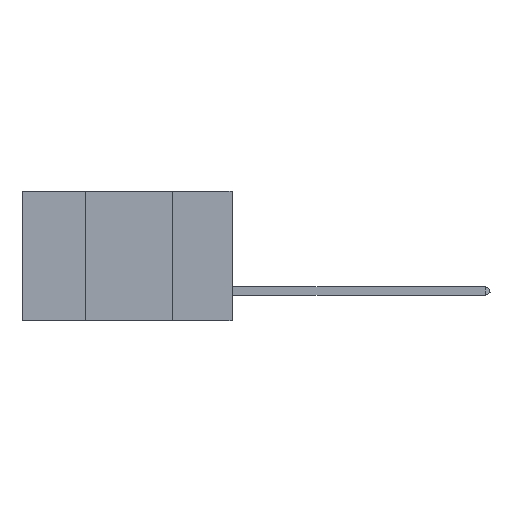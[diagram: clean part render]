
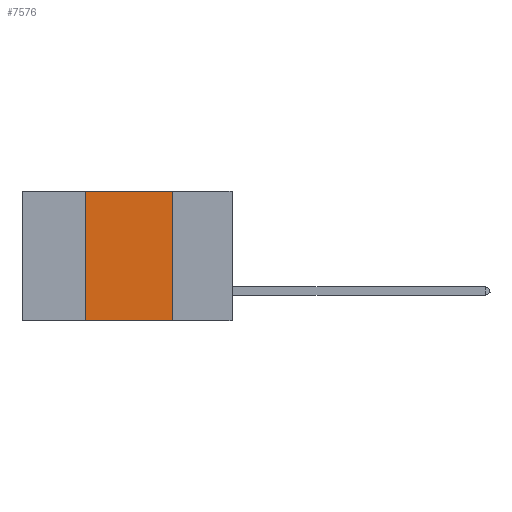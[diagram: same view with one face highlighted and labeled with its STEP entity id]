
A CAD part, left-side view. The second image highlights one B-rep face of the part: STEP entity #7576.
In plain terms, the highlighted planar face has unit normal (-1, 0, 0).
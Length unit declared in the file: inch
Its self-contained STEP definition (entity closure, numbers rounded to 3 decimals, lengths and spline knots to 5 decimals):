
#1481 = DIRECTION ( 'NONE',  ( 0., -1., 0. ) ) ;
#2502 = VECTOR ( 'NONE', #1481, 39.37008 ) ;
#2817 = AXIS2_PLACEMENT_3D ( 'NONE', #18901, #9500, #28714 ) ;
#4020 = LINE ( 'NONE', #27157, #8464 ) ;
#4046 = CARTESIAN_POINT ( 'NONE',  ( 0., 0.17, 0. ) ) ;
#4150 = EDGE_CURVE ( 'NONE', #23712, #28353, #4020, .T. ) ;
#4192 = EDGE_CURVE ( 'NONE', #16608, #23712, #28757, .T. ) ;
#5311 = CARTESIAN_POINT ( 'NONE',  ( 0., 0.6, 0. ) ) ;
#7089 = ORIENTED_EDGE ( 'NONE', *, *, #12730, .F. ) ;
#7200 = PLANE ( 'NONE',  #2817 ) ;
#7576 = ADVANCED_FACE ( 'NONE', ( #10854 ), #7200, .F. ) ;
#7782 = LINE ( 'NONE', #14104, #9268 ) ;
#8464 = VECTOR ( 'NONE', #20046, 39.37008 ) ;
#8812 = CARTESIAN_POINT ( 'NONE',  ( 0., 0.42, -0.37 ) ) ;
#9268 = VECTOR ( 'NONE', #13898, 39.37008 ) ;
#9500 = DIRECTION ( 'NONE',  ( 1., 0., 0. ) ) ;
#9719 = CARTESIAN_POINT ( 'NONE',  ( 0., 0.17, -0.37 ) ) ;
#10376 = ORIENTED_EDGE ( 'NONE', *, *, #4150, .F. ) ;
#10854 = FACE_OUTER_BOUND ( 'NONE', #30782, .T. ) ;
#12133 = DIRECTION ( 'NONE',  ( 0., -1., 0. ) ) ;
#12730 = EDGE_CURVE ( 'NONE', #28231, #16608, #7782, .T. ) ;
#13898 = DIRECTION ( 'NONE',  ( 0., 0., 1. ) ) ;
#14104 = CARTESIAN_POINT ( 'NONE',  ( 0., 0.42, 0. ) ) ;
#14160 = EDGE_CURVE ( 'NONE', #28231, #28353, #26838, .T. ) ;
#16608 = VERTEX_POINT ( 'NONE', #20420 ) ;
#18511 = CARTESIAN_POINT ( 'NONE',  ( 0., 0.6, -0.37 ) ) ;
#18901 = CARTESIAN_POINT ( 'NONE',  ( 0., 0.6, 0. ) ) ;
#20046 = DIRECTION ( 'NONE',  ( 0., 0., -1. ) ) ;
#20420 = CARTESIAN_POINT ( 'NONE',  ( 0., 0.42, 0. ) ) ;
#20495 = VECTOR ( 'NONE', #12133, 39.37008 ) ;
#21806 = ORIENTED_EDGE ( 'NONE', *, *, #14160, .T. ) ;
#23712 = VERTEX_POINT ( 'NONE', #4046 ) ;
#26167 = ORIENTED_EDGE ( 'NONE', *, *, #4192, .F. ) ;
#26838 = LINE ( 'NONE', #18511, #20495 ) ;
#27157 = CARTESIAN_POINT ( 'NONE',  ( 0., 0.17, 0. ) ) ;
#28231 = VERTEX_POINT ( 'NONE', #8812 ) ;
#28353 = VERTEX_POINT ( 'NONE', #9719 ) ;
#28714 = DIRECTION ( 'NONE',  ( 0., 0., -1. ) ) ;
#28757 = LINE ( 'NONE', #5311, #2502 ) ;
#30782 = EDGE_LOOP ( 'NONE', ( #10376, #26167, #7089, #21806 ) ) ;
